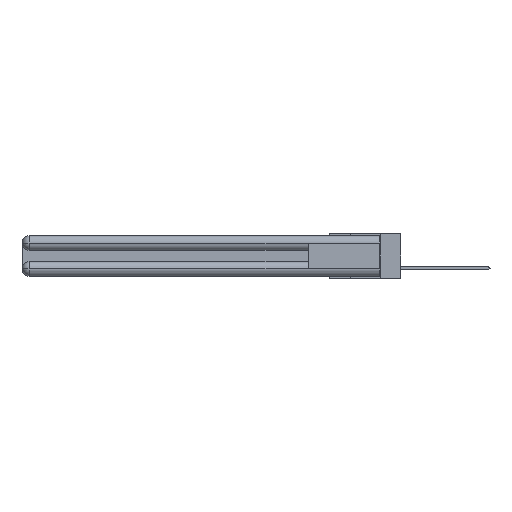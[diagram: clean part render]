
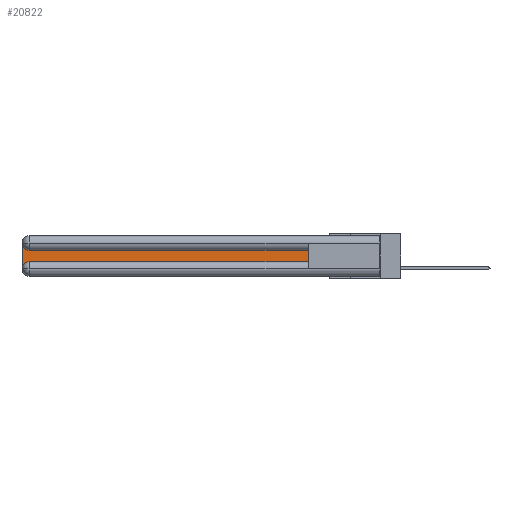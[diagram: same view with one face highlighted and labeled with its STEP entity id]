
A CAD part, left-side view. The second image highlights one B-rep face of the part: STEP entity #20822.
In plain terms, the highlighted planar face has unit normal (-1, 0, 0).
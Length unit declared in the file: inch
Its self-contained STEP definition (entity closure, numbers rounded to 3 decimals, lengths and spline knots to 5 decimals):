
#373 = VERTEX_POINT ( 'NONE', #24021 ) ;
#2012 = VERTEX_POINT ( 'NONE', #24224 ) ;
#2269 = LINE ( 'NONE', #16716, #14165 ) ;
#2768 = ORIENTED_EDGE ( 'NONE', *, *, #3679, .T. ) ;
#3240 = VECTOR ( 'NONE', #24105, 39.37008 ) ;
#3679 = EDGE_CURVE ( 'NONE', #5019, #2012, #30411, .T. ) ;
#4348 = PLANE ( 'NONE',  #9398 ) ;
#4531 = CARTESIAN_POINT ( 'NONE',  ( 0.075, 0.6, -0.2175 ) ) ;
#4654 = DIRECTION ( 'NONE',  ( 0., 0., -1. ) ) ;
#5019 = VERTEX_POINT ( 'NONE', #15010 ) ;
#5776 = AXIS2_PLACEMENT_3D ( 'NONE', #30617, #18402, #15928 ) ;
#7723 = CARTESIAN_POINT ( 'NONE',  ( 0.075, 2.94, -0.2775 ) ) ;
#9124 = LINE ( 'NONE', #22467, #21769 ) ;
#9302 = ORIENTED_EDGE ( 'NONE', *, *, #28824, .T. ) ;
#9318 = DIRECTION ( 'NONE',  ( 1., 0., 0. ) ) ;
#9398 = AXIS2_PLACEMENT_3D ( 'NONE', #16291, #9318, #4654 ) ;
#10107 = CARTESIAN_POINT ( 'NONE',  ( 0.075, 3., -0.0625 ) ) ;
#10113 = DIRECTION ( 'NONE',  ( 1., 0., 0. ) ) ;
#10249 = VERTEX_POINT ( 'NONE', #25181 ) ;
#10619 = VERTEX_POINT ( 'NONE', #10107 ) ;
#10960 = VECTOR ( 'NONE', #16767, 39.37008 ) ;
#11865 = CIRCLE ( 'NONE', #5776, 0.06 ) ;
#12898 = LINE ( 'NONE', #26289, #3240 ) ;
#14165 = VECTOR ( 'NONE', #14206, 39.37008 ) ;
#14206 = DIRECTION ( 'NONE',  ( 0., 0., 1. ) ) ;
#14294 = AXIS2_PLACEMENT_3D ( 'NONE', #7723, #10113, #15180 ) ;
#15010 = CARTESIAN_POINT ( 'NONE',  ( 0.075, 2.94, -0.2175 ) ) ;
#15180 = DIRECTION ( 'NONE',  ( 0., 0., -1. ) ) ;
#15471 = EDGE_LOOP ( 'NONE', ( #30596, #27405, #28300, #9302, #2768, #22342 ) ) ;
#15928 = DIRECTION ( 'NONE',  ( 0., 0., -1. ) ) ;
#16291 = CARTESIAN_POINT ( 'NONE',  ( 0.075, 3., -0.1225 ) ) ;
#16713 = CIRCLE ( 'NONE', #14294, 0.06 ) ;
#16716 = CARTESIAN_POINT ( 'NONE',  ( 0.075, 0.6, -0.2175 ) ) ;
#16767 = DIRECTION ( 'NONE',  ( 0., -1., 0. ) ) ;
#17294 = EDGE_CURVE ( 'NONE', #30435, #10619, #11865, .T. ) ;
#18181 = EDGE_CURVE ( 'NONE', #10619, #373, #12898, .T. ) ;
#18267 = CARTESIAN_POINT ( 'NONE',  ( 0.075, 2.94, -0.1225 ) ) ;
#18402 = DIRECTION ( 'NONE',  ( 1., 0., 0. ) ) ;
#18548 = FACE_OUTER_BOUND ( 'NONE', #15471, .T. ) ;
#19075 = EDGE_CURVE ( 'NONE', #10249, #30435, #9124, .T. ) ;
#20822 = ADVANCED_FACE ( 'NONE', ( #18548 ), #4348, .F. ) ;
#21769 = VECTOR ( 'NONE', #25096, 39.37008 ) ;
#22342 = ORIENTED_EDGE ( 'NONE', *, *, #27768, .T. ) ;
#22467 = CARTESIAN_POINT ( 'NONE',  ( 0.075, 0.6, -0.1225 ) ) ;
#24021 = CARTESIAN_POINT ( 'NONE',  ( 0.075, 3., -0.2775 ) ) ;
#24105 = DIRECTION ( 'NONE',  ( 0., 0., -1. ) ) ;
#24224 = CARTESIAN_POINT ( 'NONE',  ( 0.075, 0.6, -0.2175 ) ) ;
#25096 = DIRECTION ( 'NONE',  ( 0., 1., 0. ) ) ;
#25181 = CARTESIAN_POINT ( 'NONE',  ( 0.075, 0.6, -0.1225 ) ) ;
#26289 = CARTESIAN_POINT ( 'NONE',  ( 0.075, 3., -0.2175 ) ) ;
#27405 = ORIENTED_EDGE ( 'NONE', *, *, #17294, .T. ) ;
#27768 = EDGE_CURVE ( 'NONE', #2012, #10249, #2269, .T. ) ;
#28300 = ORIENTED_EDGE ( 'NONE', *, *, #18181, .T. ) ;
#28824 = EDGE_CURVE ( 'NONE', #373, #5019, #16713, .T. ) ;
#30411 = LINE ( 'NONE', #4531, #10960 ) ;
#30435 = VERTEX_POINT ( 'NONE', #18267 ) ;
#30596 = ORIENTED_EDGE ( 'NONE', *, *, #19075, .T. ) ;
#30617 = CARTESIAN_POINT ( 'NONE',  ( 0.075, 2.94, -0.0625 ) ) ;
